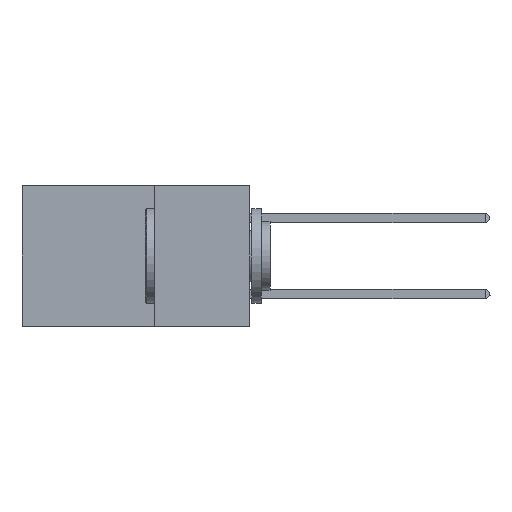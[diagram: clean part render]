
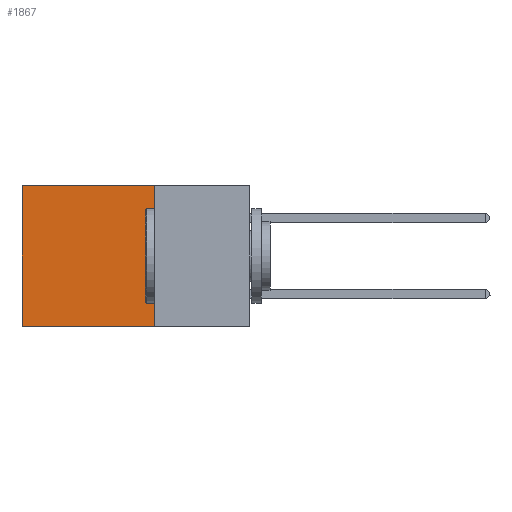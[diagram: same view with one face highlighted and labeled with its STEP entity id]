
A CAD part, left-side view. The second image highlights one B-rep face of the part: STEP entity #1867.
In plain terms, the highlighted planar face has unit normal (-1, 0, 0).
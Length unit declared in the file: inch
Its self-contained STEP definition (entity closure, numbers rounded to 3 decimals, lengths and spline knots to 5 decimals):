
#200 = VECTOR ( 'NONE', #5271, 39.37008 ) ;
#859 = VERTEX_POINT ( 'NONE', #8928 ) ;
#887 = EDGE_CURVE ( 'NONE', #859, #9063, #20940, .T. ) ;
#1831 = CARTESIAN_POINT ( 'NONE',  ( 0.2875, 0.25, -0.37 ) ) ;
#1867 = ADVANCED_FACE ( 'NONE', ( #17792 ), #9338, .F. ) ;
#2186 = VECTOR ( 'NONE', #6067, 39.37008 ) ;
#2416 = VERTEX_POINT ( 'NONE', #10812 ) ;
#3358 = VECTOR ( 'NONE', #17196, 39.37008 ) ;
#5271 = DIRECTION ( 'NONE',  ( 0., 0., -1. ) ) ;
#6067 = DIRECTION ( 'NONE',  ( 0., 1., 0. ) ) ;
#6452 = LINE ( 'NONE', #11810, #3358 ) ;
#6461 = CARTESIAN_POINT ( 'NONE',  ( 0.2875, 0.6, 0. ) ) ;
#7500 = VERTEX_POINT ( 'NONE', #6461 ) ;
#7613 = CARTESIAN_POINT ( 'NONE',  ( 0.2875, 0.25, 0. ) ) ;
#8928 = CARTESIAN_POINT ( 'NONE',  ( 0.2875, 0.25, 0. ) ) ;
#9063 = VERTEX_POINT ( 'NONE', #1831 ) ;
#9338 = PLANE ( 'NONE',  #22273 ) ;
#9409 = EDGE_CURVE ( 'NONE', #859, #7500, #16235, .T. ) ;
#10812 = CARTESIAN_POINT ( 'NONE',  ( 0.2875, 0.6, -0.37 ) ) ;
#10895 = EDGE_LOOP ( 'NONE', ( #19709, #11345, #15970, #16125 ) ) ;
#11345 = ORIENTED_EDGE ( 'NONE', *, *, #18599, .F. ) ;
#11810 = CARTESIAN_POINT ( 'NONE',  ( 0.2875, 0.25, -0.37 ) ) ;
#13121 = DIRECTION ( 'NONE',  ( 0., 0., -1. ) ) ;
#15970 = ORIENTED_EDGE ( 'NONE', *, *, #887, .F. ) ;
#16111 = CARTESIAN_POINT ( 'NONE',  ( 0.2875, 0.25, 0. ) ) ;
#16125 = ORIENTED_EDGE ( 'NONE', *, *, #9409, .T. ) ;
#16235 = LINE ( 'NONE', #16111, #2186 ) ;
#17196 = DIRECTION ( 'NONE',  ( 0., 1., 0. ) ) ;
#17792 = FACE_OUTER_BOUND ( 'NONE', #10895, .T. ) ;
#17881 = DIRECTION ( 'NONE',  ( 0., 0., -1. ) ) ;
#18422 = DIRECTION ( 'NONE',  ( 1., 0., 0. ) ) ;
#18599 = EDGE_CURVE ( 'NONE', #9063, #2416, #6452, .T. ) ;
#19480 = CARTESIAN_POINT ( 'NONE',  ( 0.2875, 0.6, 0. ) ) ;
#19491 = EDGE_CURVE ( 'NONE', #7500, #2416, #20757, .T. ) ;
#19709 = ORIENTED_EDGE ( 'NONE', *, *, #19491, .T. ) ;
#20757 = LINE ( 'NONE', #19480, #200 ) ;
#20940 = LINE ( 'NONE', #23092, #22307 ) ;
#22273 = AXIS2_PLACEMENT_3D ( 'NONE', #7613, #18422, #13121 ) ;
#22307 = VECTOR ( 'NONE', #17881, 39.37008 ) ;
#23092 = CARTESIAN_POINT ( 'NONE',  ( 0.2875, 0.25, 0. ) ) ;
